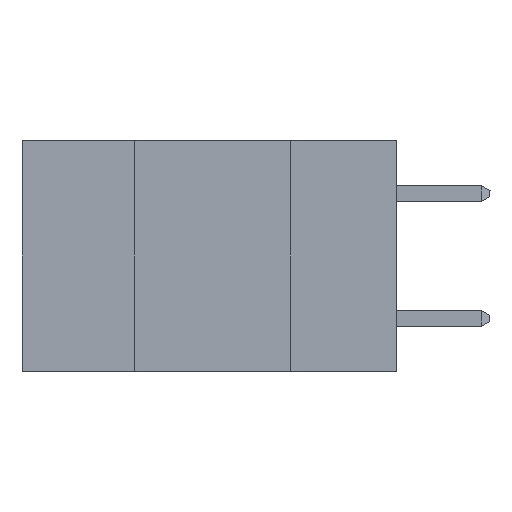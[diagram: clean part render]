
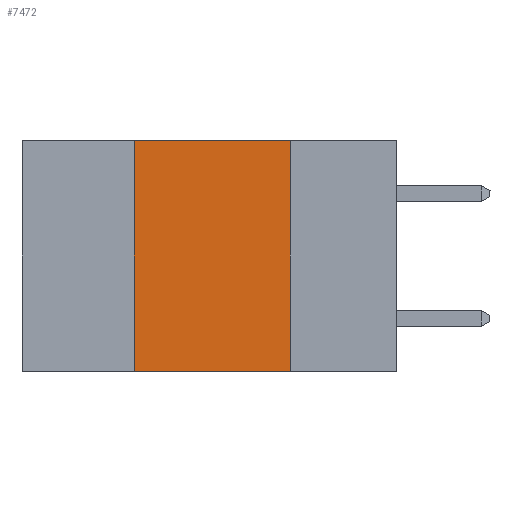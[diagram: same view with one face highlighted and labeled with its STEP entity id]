
A CAD part, left-side view. The second image highlights one B-rep face of the part: STEP entity #7472.
In plain terms, the highlighted planar face has unit normal (-1, 0, 0).
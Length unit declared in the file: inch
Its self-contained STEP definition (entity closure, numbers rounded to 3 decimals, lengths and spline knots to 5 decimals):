
#1065 = DIRECTION ( 'NONE',  ( 0., -1., 0. ) ) ;
#1949 = EDGE_CURVE ( 'NONE', #4441, #3050, #7361, .T. ) ;
#2605 = EDGE_CURVE ( 'NONE', #3050, #12315, #6020, .T. ) ;
#2921 = VECTOR ( 'NONE', #11005, 39.37008 ) ;
#3050 = VERTEX_POINT ( 'NONE', #7741 ) ;
#3766 = DIRECTION ( 'NONE',  ( 0., 0., 1. ) ) ;
#4429 = ORIENTED_EDGE ( 'NONE', *, *, #1949, .F. ) ;
#4441 = VERTEX_POINT ( 'NONE', #7167 ) ;
#5875 = AXIS2_PLACEMENT_3D ( 'NONE', #19065, #18926, #18768 ) ;
#6020 = LINE ( 'NONE', #15664, #18366 ) ;
#6440 = EDGE_LOOP ( 'NONE', ( #14013, #4429, #9366, #17868 ) ) ;
#6824 = VECTOR ( 'NONE', #1065, 39.37008 ) ;
#7167 = CARTESIAN_POINT ( 'NONE',  ( 0., 0.42, 0. ) ) ;
#7361 = LINE ( 'NONE', #15502, #6824 ) ;
#7420 = LINE ( 'NONE', #14225, #2921 ) ;
#7472 = ADVANCED_FACE ( 'NONE', ( #13587 ), #19193, .F. ) ;
#7634 = CARTESIAN_POINT ( 'NONE',  ( 0., 0.42, -0.37 ) ) ;
#7741 = CARTESIAN_POINT ( 'NONE',  ( 0., 0.17, 0. ) ) ;
#9366 = ORIENTED_EDGE ( 'NONE', *, *, #20388, .F. ) ;
#9569 = CARTESIAN_POINT ( 'NONE',  ( 0., 0.17, -0.37 ) ) ;
#9974 = DIRECTION ( 'NONE',  ( 0., 0., -1. ) ) ;
#11005 = DIRECTION ( 'NONE',  ( 0., -1., 0. ) ) ;
#12315 = VERTEX_POINT ( 'NONE', #9569 ) ;
#12937 = EDGE_CURVE ( 'NONE', #14806, #12315, #7420, .T. ) ;
#13587 = FACE_OUTER_BOUND ( 'NONE', #6440, .T. ) ;
#14013 = ORIENTED_EDGE ( 'NONE', *, *, #2605, .F. ) ;
#14102 = VECTOR ( 'NONE', #3766, 39.37008 ) ;
#14225 = CARTESIAN_POINT ( 'NONE',  ( 0., 0.6, -0.37 ) ) ;
#14806 = VERTEX_POINT ( 'NONE', #7634 ) ;
#15502 = CARTESIAN_POINT ( 'NONE',  ( 0., 0.6, 0. ) ) ;
#15664 = CARTESIAN_POINT ( 'NONE',  ( 0., 0.17, 0. ) ) ;
#17868 = ORIENTED_EDGE ( 'NONE', *, *, #12937, .T. ) ;
#18361 = LINE ( 'NONE', #19904, #14102 ) ;
#18366 = VECTOR ( 'NONE', #9974, 39.37008 ) ;
#18768 = DIRECTION ( 'NONE',  ( 0., 0., -1. ) ) ;
#18926 = DIRECTION ( 'NONE',  ( 1., 0., 0. ) ) ;
#19065 = CARTESIAN_POINT ( 'NONE',  ( 0., 0.6, 0. ) ) ;
#19193 = PLANE ( 'NONE',  #5875 ) ;
#19904 = CARTESIAN_POINT ( 'NONE',  ( 0., 0.42, 0. ) ) ;
#20388 = EDGE_CURVE ( 'NONE', #14806, #4441, #18361, .T. ) ;
